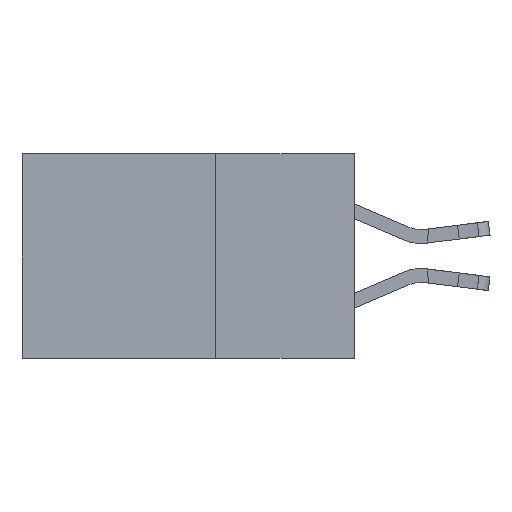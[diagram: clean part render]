
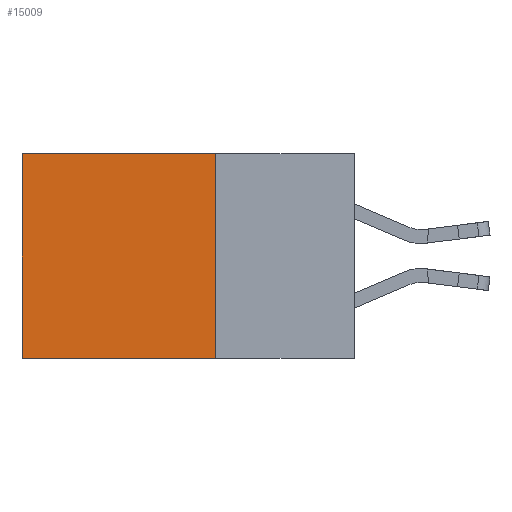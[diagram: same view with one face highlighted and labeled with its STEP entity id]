
A CAD part, left-side view. The second image highlights one B-rep face of the part: STEP entity #15009.
In plain terms, the highlighted planar face has unit normal (-1, 0, 0).
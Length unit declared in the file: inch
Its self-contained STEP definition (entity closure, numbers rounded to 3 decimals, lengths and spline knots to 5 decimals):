
#794 = EDGE_CURVE ( 'NONE', #9834, #21316, #16948, .T. ) ;
#1029 = DIRECTION ( 'NONE',  ( 0., 0., -1. ) ) ;
#1429 = VECTOR ( 'NONE', #17378, 39.37008 ) ;
#1438 = CARTESIAN_POINT ( 'NONE',  ( 0.2615, 0.6, -0.37 ) ) ;
#1841 = DIRECTION ( 'NONE',  ( 0., 0., -1. ) ) ;
#2235 = VECTOR ( 'NONE', #1029, 39.37008 ) ;
#3206 = CARTESIAN_POINT ( 'NONE',  ( 0.2615, 0.25, -0.37 ) ) ;
#3276 = DIRECTION ( 'NONE',  ( 0., 1., 0. ) ) ;
#4754 = CARTESIAN_POINT ( 'NONE',  ( 0.2615, 0.25, -0.37 ) ) ;
#5495 = ORIENTED_EDGE ( 'NONE', *, *, #22950, .F. ) ;
#5985 = LINE ( 'NONE', #9457, #1429 ) ;
#6539 = PLANE ( 'NONE',  #13182 ) ;
#7070 = VERTEX_POINT ( 'NONE', #3206 ) ;
#7380 = ORIENTED_EDGE ( 'NONE', *, *, #18268, .T. ) ;
#7521 = VECTOR ( 'NONE', #3276, 39.37008 ) ;
#9086 = LINE ( 'NONE', #20229, #7521 ) ;
#9399 = CARTESIAN_POINT ( 'NONE',  ( 0.2615, 0.6, -0.37 ) ) ;
#9457 = CARTESIAN_POINT ( 'NONE',  ( 0.2615, 0.25, 0. ) ) ;
#9732 = EDGE_LOOP ( 'NONE', ( #20899, #5495, #13838, #7380 ) ) ;
#9834 = VERTEX_POINT ( 'NONE', #11643 ) ;
#10287 = VECTOR ( 'NONE', #1841, 39.37008 ) ;
#11643 = CARTESIAN_POINT ( 'NONE',  ( 0.2615, 0.6, 0. ) ) ;
#12314 = LINE ( 'NONE', #4754, #2235 ) ;
#13182 = AXIS2_PLACEMENT_3D ( 'NONE', #15976, #14114, #14238 ) ;
#13838 = ORIENTED_EDGE ( 'NONE', *, *, #18371, .F. ) ;
#14114 = DIRECTION ( 'NONE',  ( 1., 0., 0. ) ) ;
#14238 = DIRECTION ( 'NONE',  ( 0., 0., -1. ) ) ;
#15009 = ADVANCED_FACE ( 'NONE', ( #15728 ), #6539, .F. ) ;
#15728 = FACE_OUTER_BOUND ( 'NONE', #9732, .T. ) ;
#15976 = CARTESIAN_POINT ( 'NONE',  ( 0.2615, 0.25, -0.37 ) ) ;
#16948 = LINE ( 'NONE', #9399, #10287 ) ;
#17378 = DIRECTION ( 'NONE',  ( 0., 1., 0. ) ) ;
#17900 = CARTESIAN_POINT ( 'NONE',  ( 0.2615, 0.25, 0. ) ) ;
#17931 = VERTEX_POINT ( 'NONE', #17900 ) ;
#18268 = EDGE_CURVE ( 'NONE', #17931, #9834, #5985, .T. ) ;
#18371 = EDGE_CURVE ( 'NONE', #17931, #7070, #12314, .T. ) ;
#20229 = CARTESIAN_POINT ( 'NONE',  ( 0.2615, 0.25, -0.37 ) ) ;
#20899 = ORIENTED_EDGE ( 'NONE', *, *, #794, .T. ) ;
#21316 = VERTEX_POINT ( 'NONE', #1438 ) ;
#22950 = EDGE_CURVE ( 'NONE', #7070, #21316, #9086, .T. ) ;
